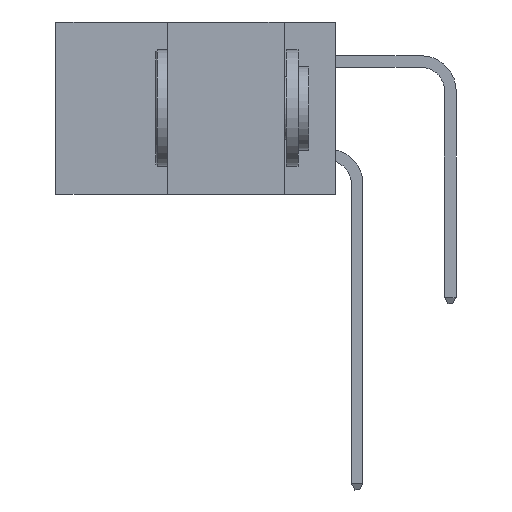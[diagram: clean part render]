
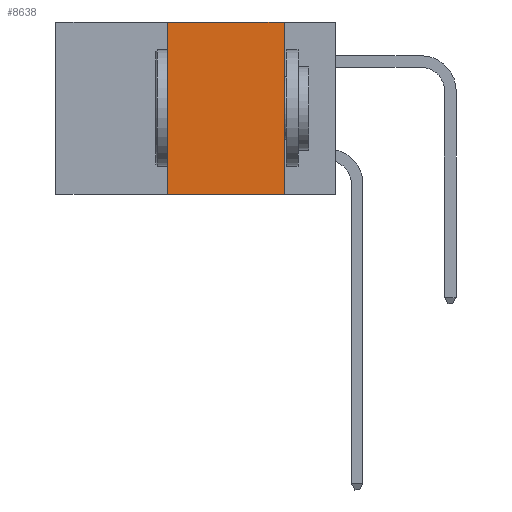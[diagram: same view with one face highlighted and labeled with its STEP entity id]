
A CAD part, left-side view. The second image highlights one B-rep face of the part: STEP entity #8638.
In plain terms, the highlighted planar face has unit normal (-1, 0, 0).
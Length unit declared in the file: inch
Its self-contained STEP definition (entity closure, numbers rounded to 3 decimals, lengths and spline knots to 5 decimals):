
#384 = CARTESIAN_POINT ( 'NONE',  ( 0., 0.36, 0. ) ) ;
#1617 = AXIS2_PLACEMENT_3D ( 'NONE', #2704, #14571, #4377 ) ;
#2704 = CARTESIAN_POINT ( 'NONE',  ( 0., 0.6, 0. ) ) ;
#3207 = DIRECTION ( 'NONE',  ( 0., 0., 1. ) ) ;
#3866 = LINE ( 'NONE', #14815, #21127 ) ;
#4287 = EDGE_CURVE ( 'NONE', #12508, #5377, #3866, .T. ) ;
#4377 = DIRECTION ( 'NONE',  ( 0., 0., -1. ) ) ;
#4589 = VECTOR ( 'NONE', #3207, 39.37008 ) ;
#5377 = VERTEX_POINT ( 'NONE', #13155 ) ;
#6545 = CARTESIAN_POINT ( 'NONE',  ( 0., 0.6, 0. ) ) ;
#7801 = VERTEX_POINT ( 'NONE', #8690 ) ;
#7818 = EDGE_CURVE ( 'NONE', #7801, #5377, #13885, .T. ) ;
#7886 = VERTEX_POINT ( 'NONE', #384 ) ;
#8638 = ADVANCED_FACE ( 'NONE', ( #15386 ), #12906, .F. ) ;
#8690 = CARTESIAN_POINT ( 'NONE',  ( 0., 0.11, 0. ) ) ;
#9399 = VECTOR ( 'NONE', #13833, 39.37008 ) ;
#9755 = VECTOR ( 'NONE', #16549, 39.37008 ) ;
#10642 = EDGE_CURVE ( 'NONE', #7886, #7801, #18538, .T. ) ;
#12196 = EDGE_LOOP ( 'NONE', ( #13954, #14191, #14342, #14452 ) ) ;
#12324 = EDGE_CURVE ( 'NONE', #12508, #7886, #21318, .T. ) ;
#12508 = VERTEX_POINT ( 'NONE', #14059 ) ;
#12906 = PLANE ( 'NONE',  #1617 ) ;
#13155 = CARTESIAN_POINT ( 'NONE',  ( 0., 0.11, -0.37 ) ) ;
#13833 = DIRECTION ( 'NONE',  ( 0., 0., -1. ) ) ;
#13885 = LINE ( 'NONE', #18653, #9399 ) ;
#13954 = ORIENTED_EDGE ( 'NONE', *, *, #7818, .F. ) ;
#14059 = CARTESIAN_POINT ( 'NONE',  ( 0., 0.36, -0.37 ) ) ;
#14191 = ORIENTED_EDGE ( 'NONE', *, *, #10642, .F. ) ;
#14342 = ORIENTED_EDGE ( 'NONE', *, *, #12324, .F. ) ;
#14452 = ORIENTED_EDGE ( 'NONE', *, *, #4287, .T. ) ;
#14571 = DIRECTION ( 'NONE',  ( 1., 0., 0. ) ) ;
#14815 = CARTESIAN_POINT ( 'NONE',  ( 0., 0.6, -0.37 ) ) ;
#15077 = CARTESIAN_POINT ( 'NONE',  ( 0., 0.36, 0. ) ) ;
#15386 = FACE_OUTER_BOUND ( 'NONE', #12196, .T. ) ;
#16549 = DIRECTION ( 'NONE',  ( 0., -1., 0. ) ) ;
#18274 = DIRECTION ( 'NONE',  ( 0., -1., 0. ) ) ;
#18538 = LINE ( 'NONE', #6545, #9755 ) ;
#18653 = CARTESIAN_POINT ( 'NONE',  ( 0., 0.11, 0. ) ) ;
#21127 = VECTOR ( 'NONE', #18274, 39.37008 ) ;
#21318 = LINE ( 'NONE', #15077, #4589 ) ;
